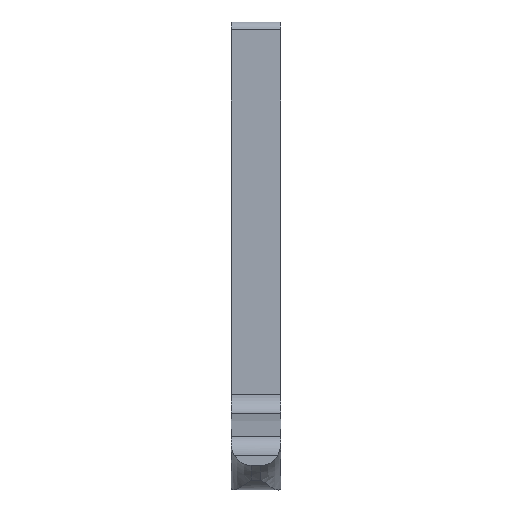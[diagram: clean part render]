
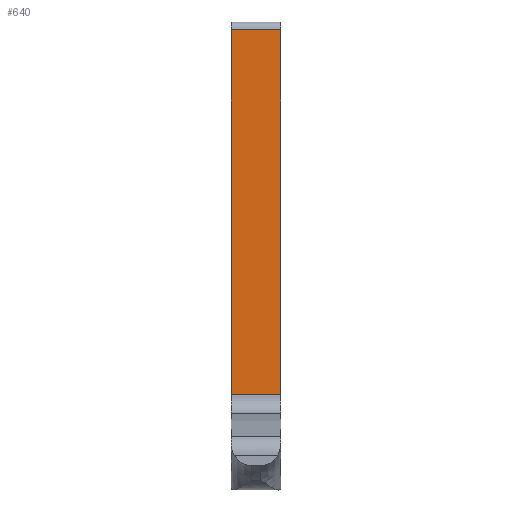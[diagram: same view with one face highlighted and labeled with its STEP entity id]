
A CAD part, front view. The second image highlights one B-rep face of the part: STEP entity #640.
In plain terms, the highlighted planar face has unit normal (0, -1, 0).
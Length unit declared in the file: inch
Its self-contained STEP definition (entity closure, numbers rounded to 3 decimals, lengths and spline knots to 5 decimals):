
#1 = DIRECTION ( 'NONE',  ( -1., 0., 0. ) ) ;
#10 = CARTESIAN_POINT ( 'NONE',  ( 0.25, 0., 0.2972 ) ) ;
#26 = LINE ( 'NONE', #591, #1008 ) ;
#86 = CARTESIAN_POINT ( 'NONE',  ( 0.25, 0., 0.2972 ) ) ;
#150 = ORIENTED_EDGE ( 'NONE', *, *, #897, .T. ) ;
#190 = DIRECTION ( 'NONE',  ( 0., 1., 0. ) ) ;
#214 = DIRECTION ( 'NONE',  ( 0., 0., -1. ) ) ;
#231 = VERTEX_POINT ( 'NONE', #10 ) ;
#238 = CARTESIAN_POINT ( 'NONE',  ( 0., 0., 0.2972 ) ) ;
#288 = VECTOR ( 'NONE', #940, 39.37008 ) ;
#292 = LINE ( 'NONE', #378, #985 ) ;
#372 = VERTEX_POINT ( 'NONE', #238 ) ;
#378 = CARTESIAN_POINT ( 'NONE',  ( 0.25, 0., 2.1475 ) ) ;
#526 = LINE ( 'NONE', #86, #288 ) ;
#560 = CARTESIAN_POINT ( 'NONE',  ( 0.25, 0., 0.1875 ) ) ;
#568 = CARTESIAN_POINT ( 'NONE',  ( 0., 0., 0.1875 ) ) ;
#574 = CARTESIAN_POINT ( 'NONE',  ( 0.25, 0., 2.1475 ) ) ;
#591 = CARTESIAN_POINT ( 'NONE',  ( 0.25, 0., 0.1875 ) ) ;
#640 = ADVANCED_FACE ( 'NONE', ( #718 ), #1123, .F. ) ;
#656 = VECTOR ( 'NONE', #768, 39.37008 ) ;
#696 = EDGE_CURVE ( 'NONE', #928, #372, #1155, .T. ) ;
#718 = FACE_OUTER_BOUND ( 'NONE', #861, .T. ) ;
#757 = AXIS2_PLACEMENT_3D ( 'NONE', #560, #190, #859 ) ;
#768 = DIRECTION ( 'NONE',  ( 0., 0., -1. ) ) ;
#830 = ORIENTED_EDGE ( 'NONE', *, *, #1082, .T. ) ;
#834 = ORIENTED_EDGE ( 'NONE', *, *, #1187, .F. ) ;
#852 = CARTESIAN_POINT ( 'NONE',  ( 0., 0., 2.1475 ) ) ;
#859 = DIRECTION ( 'NONE',  ( 0., 0., 1. ) ) ;
#861 = EDGE_LOOP ( 'NONE', ( #934, #150, #834, #830 ) ) ;
#897 = EDGE_CURVE ( 'NONE', #372, #231, #526, .T. ) ;
#928 = VERTEX_POINT ( 'NONE', #852 ) ;
#934 = ORIENTED_EDGE ( 'NONE', *, *, #696, .T. ) ;
#940 = DIRECTION ( 'NONE',  ( 1., 0., 0. ) ) ;
#985 = VECTOR ( 'NONE', #1, 39.37008 ) ;
#1008 = VECTOR ( 'NONE', #214, 39.37008 ) ;
#1082 = EDGE_CURVE ( 'NONE', #1089, #928, #292, .T. ) ;
#1089 = VERTEX_POINT ( 'NONE', #574 ) ;
#1123 = PLANE ( 'NONE',  #757 ) ;
#1155 = LINE ( 'NONE', #568, #656 ) ;
#1187 = EDGE_CURVE ( 'NONE', #1089, #231, #26, .T. ) ;
